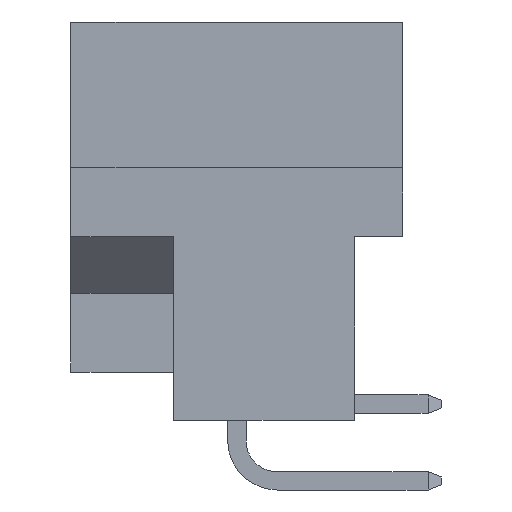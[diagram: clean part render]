
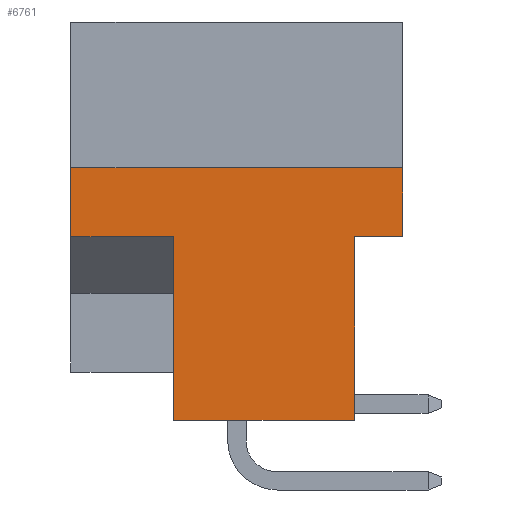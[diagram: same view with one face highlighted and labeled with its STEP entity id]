
A CAD part, left-side view. The second image highlights one B-rep face of the part: STEP entity #6761.
In plain terms, the highlighted planar face has unit normal (-1, 0, 0).
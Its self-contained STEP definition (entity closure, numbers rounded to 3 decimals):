
#71 = DIRECTION ( 'NONE',  ( 0., 0., 1. ) ) ;
#367 = CARTESIAN_POINT ( 'NONE',  ( 0., 10.998, -4.826 ) ) ;
#561 = ORIENTED_EDGE ( 'NONE', *, *, #10700, .F. ) ;
#681 = VERTEX_POINT ( 'NONE', #12552 ) ;
#794 = LINE ( 'NONE', #13441, #7122 ) ;
#1439 = VECTOR ( 'NONE', #7268, 1000. ) ;
#1625 = CARTESIAN_POINT ( 'NONE',  ( 0., 0., -4.826 ) ) ;
#2037 = EDGE_CURVE ( 'NONE', #5342, #4697, #16107, .T. ) ;
#2257 = ORIENTED_EDGE ( 'NONE', *, *, #9968, .F. ) ;
#2394 = ORIENTED_EDGE ( 'NONE', *, *, #4248, .F. ) ;
#2649 = CARTESIAN_POINT ( 'NONE',  ( 0., 10.998, 0. ) ) ;
#2797 = CARTESIAN_POINT ( 'NONE',  ( 0., 1.6, -7.112 ) ) ;
#2980 = FACE_OUTER_BOUND ( 'NONE', #4643, .T. ) ;
#3266 = ORIENTED_EDGE ( 'NONE', *, *, #15628, .F. ) ;
#3515 = DIRECTION ( 'NONE',  ( 0., 0., 1. ) ) ;
#3930 = VECTOR ( 'NONE', #11190, 1000. ) ;
#4248 = EDGE_CURVE ( 'NONE', #681, #7514, #15164, .T. ) ;
#4434 = VECTOR ( 'NONE', #14620, 1000. ) ;
#4643 = EDGE_LOOP ( 'NONE', ( #6807, #9472, #5837, #561, #3266, #2257, #2394, #8271 ) ) ;
#4697 = VERTEX_POINT ( 'NONE', #12949 ) ;
#5053 = CARTESIAN_POINT ( 'NONE',  ( 0., 0., -7.112 ) ) ;
#5097 = LINE ( 'NONE', #2649, #3930 ) ;
#5342 = VERTEX_POINT ( 'NONE', #2797 ) ;
#5518 = DIRECTION ( 'NONE',  ( 0., 0., -1. ) ) ;
#5837 = ORIENTED_EDGE ( 'NONE', *, *, #13309, .T. ) ;
#6108 = VERTEX_POINT ( 'NONE', #5053 ) ;
#6174 = CARTESIAN_POINT ( 'NONE',  ( 0., 1.6, 86.902 ) ) ;
#6380 = CARTESIAN_POINT ( 'NONE',  ( 0., 7.597, -13.2 ) ) ;
#6742 = PLANE ( 'NONE',  #7355 ) ;
#6761 = ADVANCED_FACE ( 'NONE', ( #2980 ), #6742, .F. ) ;
#6807 = ORIENTED_EDGE ( 'NONE', *, *, #2037, .F. ) ;
#7122 = VECTOR ( 'NONE', #3515, 1000. ) ;
#7268 = DIRECTION ( 'NONE',  ( 0., -1., 0. ) ) ;
#7355 = AXIS2_PLACEMENT_3D ( 'NONE', #9060, #14053, #5518 ) ;
#7438 = LINE ( 'NONE', #12444, #14817 ) ;
#7514 = VERTEX_POINT ( 'NONE', #10078 ) ;
#8271 = ORIENTED_EDGE ( 'NONE', *, *, #10723, .T. ) ;
#9060 = CARTESIAN_POINT ( 'NONE',  ( 0., 10.998, 0. ) ) ;
#9472 = ORIENTED_EDGE ( 'NONE', *, *, #15895, .F. ) ;
#9661 = DIRECTION ( 'NONE',  ( 0., -1., 0. ) ) ;
#9880 = DIRECTION ( 'NONE',  ( 0., 0., -1. ) ) ;
#9968 = EDGE_CURVE ( 'NONE', #7514, #13395, #14178, .T. ) ;
#10078 = CARTESIAN_POINT ( 'NONE',  ( 0., 7.597, -7.112 ) ) ;
#10123 = DIRECTION ( 'NONE',  ( 0., 1., 0. ) ) ;
#10689 = VECTOR ( 'NONE', #9880, 1000. ) ;
#10700 = EDGE_CURVE ( 'NONE', #10813, #13154, #13436, .T. ) ;
#10723 = EDGE_CURVE ( 'NONE', #681, #4697, #7438, .T. ) ;
#10813 = VERTEX_POINT ( 'NONE', #367 ) ;
#11067 = CARTESIAN_POINT ( 'NONE',  ( 0., 10.998, -7.112 ) ) ;
#11190 = DIRECTION ( 'NONE',  ( 0., 0., 1. ) ) ;
#12444 = CARTESIAN_POINT ( 'NONE',  ( 0., 10.998, -13.2 ) ) ;
#12445 = VECTOR ( 'NONE', #10123, 1000. ) ;
#12552 = CARTESIAN_POINT ( 'NONE',  ( 0., 7.597, -13.2 ) ) ;
#12817 = CARTESIAN_POINT ( 'NONE',  ( 0., 7.597, -7.112 ) ) ;
#12949 = CARTESIAN_POINT ( 'NONE',  ( 0., 1.6, -13.2 ) ) ;
#13154 = VERTEX_POINT ( 'NONE', #1625 ) ;
#13309 = EDGE_CURVE ( 'NONE', #6108, #13154, #794, .T. ) ;
#13395 = VERTEX_POINT ( 'NONE', #11067 ) ;
#13436 = LINE ( 'NONE', #15970, #1439 ) ;
#13441 = CARTESIAN_POINT ( 'NONE',  ( 0., 0., 0. ) ) ;
#14053 = DIRECTION ( 'NONE',  ( 1., 0., 0. ) ) ;
#14178 = LINE ( 'NONE', #12817, #12445 ) ;
#14449 = CARTESIAN_POINT ( 'NONE',  ( 0., 0., -7.112 ) ) ;
#14620 = DIRECTION ( 'NONE',  ( 0., 1., 0. ) ) ;
#14817 = VECTOR ( 'NONE', #9661, 1000. ) ;
#15063 = VECTOR ( 'NONE', #71, 1000. ) ;
#15164 = LINE ( 'NONE', #6380, #15063 ) ;
#15628 = EDGE_CURVE ( 'NONE', #13395, #10813, #5097, .T. ) ;
#15758 = LINE ( 'NONE', #14449, #4434 ) ;
#15895 = EDGE_CURVE ( 'NONE', #6108, #5342, #15758, .T. ) ;
#15970 = CARTESIAN_POINT ( 'NONE',  ( 0., 10.998, -4.826 ) ) ;
#16107 = LINE ( 'NONE', #6174, #10689 ) ;
